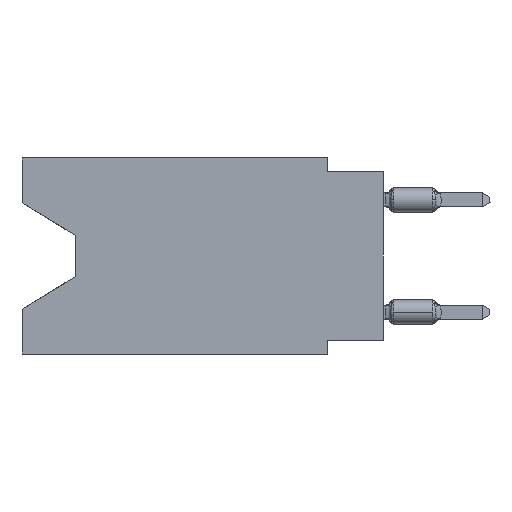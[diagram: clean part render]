
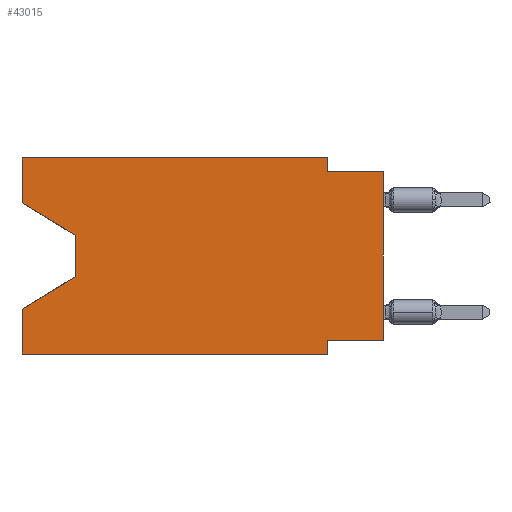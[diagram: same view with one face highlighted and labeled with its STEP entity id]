
A CAD part, left-side view. The second image highlights one B-rep face of the part: STEP entity #43015.
In plain terms, the highlighted planar face has unit normal (-1, 0, 0).
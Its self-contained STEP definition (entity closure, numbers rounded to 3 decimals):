
#37 = VERTEX_POINT ( 'NONE', #25711 ) ;
#702 = CARTESIAN_POINT ( 'NONE',  ( 0., 0., -8.255 ) ) ;
#1206 = EDGE_CURVE ( 'NONE', #21549, #45373, #19123, .T. ) ;
#2084 = PLANE ( 'NONE',  #38290 ) ;
#3101 = EDGE_CURVE ( 'NONE', #45373, #39737, #10770, .T. ) ;
#3219 = CARTESIAN_POINT ( 'NONE',  ( 0., 0., 0. ) ) ;
#4158 = CARTESIAN_POINT ( 'NONE',  ( 0., 16.383, -8.89 ) ) ;
#5878 = ORIENTED_EDGE ( 'NONE', *, *, #19402, .F. ) ;
#6076 = CARTESIAN_POINT ( 'NONE',  ( 0., 0., -0.635 ) ) ;
#7157 = ORIENTED_EDGE ( 'NONE', *, *, #35518, .T. ) ;
#7314 = CARTESIAN_POINT ( 'NONE',  ( 0., 16.383, 0. ) ) ;
#7363 = VECTOR ( 'NONE', #28769, 1000. ) ;
#8396 = DIRECTION ( 'NONE',  ( 0., 1., 0. ) ) ;
#8621 = LINE ( 'NONE', #32381, #10604 ) ;
#9791 = VECTOR ( 'NONE', #45495, 1000. ) ;
#9965 = DIRECTION ( 'NONE',  ( 0., -1., 0. ) ) ;
#10604 = VECTOR ( 'NONE', #8396, 1000. ) ;
#10770 = LINE ( 'NONE', #7314, #21943 ) ;
#11464 = EDGE_CURVE ( 'NONE', #42902, #37655, #41556, .T. ) ;
#12066 = ORIENTED_EDGE ( 'NONE', *, *, #20796, .T. ) ;
#12552 = VERTEX_POINT ( 'NONE', #20235 ) ;
#12775 = VECTOR ( 'NONE', #9965, 1000. ) ;
#13725 = LINE ( 'NONE', #44629, #23203 ) ;
#13886 = ORIENTED_EDGE ( 'NONE', *, *, #19616, .F. ) ;
#14100 = CARTESIAN_POINT ( 'NONE',  ( 0., 2.54, -8.255 ) ) ;
#14379 = ORIENTED_EDGE ( 'NONE', *, *, #3101, .F. ) ;
#14583 = DIRECTION ( 'NONE',  ( 0., 0., -1. ) ) ;
#15799 = LINE ( 'NONE', #19950, #31685 ) ;
#16766 = VECTOR ( 'NONE', #27996, 1000. ) ;
#17135 = CARTESIAN_POINT ( 'NONE',  ( 0., 2.54, -0.635 ) ) ;
#17809 = CARTESIAN_POINT ( 'NONE',  ( 0., 16.383, -8.89 ) ) ;
#18861 = CARTESIAN_POINT ( 'NONE',  ( 0., 16.383, -2.038 ) ) ;
#19123 = LINE ( 'NONE', #21899, #45384 ) ;
#19136 = FACE_OUTER_BOUND ( 'NONE', #28812, .T. ) ;
#19402 = EDGE_CURVE ( 'NONE', #19554, #37, #30507, .T. ) ;
#19421 = CARTESIAN_POINT ( 'NONE',  ( 0., 16.383, -6.852 ) ) ;
#19554 = VERTEX_POINT ( 'NONE', #17135 ) ;
#19589 = CARTESIAN_POINT ( 'NONE',  ( 0., 16.383, 0. ) ) ;
#19616 = EDGE_CURVE ( 'NONE', #24701, #37655, #31420, .T. ) ;
#19875 = VERTEX_POINT ( 'NONE', #19421 ) ;
#19950 = CARTESIAN_POINT ( 'NONE',  ( 0., 2.54, 0. ) ) ;
#20235 = CARTESIAN_POINT ( 'NONE',  ( 0., 13.97, -5.385 ) ) ;
#20460 = EDGE_CURVE ( 'NONE', #30813, #24701, #8621, .T. ) ;
#20515 = LINE ( 'NONE', #3219, #26994 ) ;
#20522 = ORIENTED_EDGE ( 'NONE', *, *, #22407, .T. ) ;
#20660 = CARTESIAN_POINT ( 'NONE',  ( 0., 16.383, -2.038 ) ) ;
#20796 = EDGE_CURVE ( 'NONE', #35473, #12552, #35106, .T. ) ;
#21198 = DIRECTION ( 'NONE',  ( 0., 0., 1. ) ) ;
#21534 = EDGE_CURVE ( 'NONE', #12552, #19875, #13725, .T. ) ;
#21549 = VERTEX_POINT ( 'NONE', #20660 ) ;
#21772 = CARTESIAN_POINT ( 'NONE',  ( 0., 16.383, 0. ) ) ;
#21899 = CARTESIAN_POINT ( 'NONE',  ( 0., 16.383, 0. ) ) ;
#21943 = VECTOR ( 'NONE', #42594, 1000. ) ;
#22407 = EDGE_CURVE ( 'NONE', #21549, #35473, #39629, .T. ) ;
#23049 = EDGE_CURVE ( 'NONE', #39737, #19554, #15799, .T. ) ;
#23203 = VECTOR ( 'NONE', #34251, 1000. ) ;
#24701 = VERTEX_POINT ( 'NONE', #14100 ) ;
#25711 = CARTESIAN_POINT ( 'NONE',  ( 0., 0., -0.635 ) ) ;
#26224 = CARTESIAN_POINT ( 'NONE',  ( 0., 2.54, 0. ) ) ;
#26994 = VECTOR ( 'NONE', #21198, 1000. ) ;
#27373 = ORIENTED_EDGE ( 'NONE', *, *, #21534, .T. ) ;
#27996 = DIRECTION ( 'NONE',  ( 0., 0., 1. ) ) ;
#28174 = CARTESIAN_POINT ( 'NONE',  ( 0., 13.97, -3.505 ) ) ;
#28769 = DIRECTION ( 'NONE',  ( 0., -0.855, -0.519 ) ) ;
#28812 = EDGE_LOOP ( 'NONE', ( #20522, #12066, #27373, #37714, #35140, #13886, #36072, #7157, #5878, #37932, #14379, #31043 ) ) ;
#29260 = DIRECTION ( 'NONE',  ( 0., 0., 1. ) ) ;
#29732 = VECTOR ( 'NONE', #14583, 1000. ) ;
#30182 = DIRECTION ( 'NONE',  ( 0., 0., -1. ) ) ;
#30507 = LINE ( 'NONE', #6076, #41454 ) ;
#30813 = VERTEX_POINT ( 'NONE', #702 ) ;
#31043 = ORIENTED_EDGE ( 'NONE', *, *, #1206, .F. ) ;
#31420 = LINE ( 'NONE', #39266, #9791 ) ;
#31685 = VECTOR ( 'NONE', #34005, 1000. ) ;
#31907 = CARTESIAN_POINT ( 'NONE',  ( 0., 2.54, -8.89 ) ) ;
#32381 = CARTESIAN_POINT ( 'NONE',  ( 0., 0., -8.255 ) ) ;
#33194 = DIRECTION ( 'NONE',  ( 1., 0., 0. ) ) ;
#33208 = CARTESIAN_POINT ( 'NONE',  ( 0., 16.383, 0. ) ) ;
#33900 = CARTESIAN_POINT ( 'NONE',  ( 0., 13.97, -3.505 ) ) ;
#34005 = DIRECTION ( 'NONE',  ( 0., 0., -1. ) ) ;
#34210 = DIRECTION ( 'NONE',  ( 0., -1., 0. ) ) ;
#34251 = DIRECTION ( 'NONE',  ( 0., 0.855, -0.519 ) ) ;
#35106 = LINE ( 'NONE', #28174, #29732 ) ;
#35140 = ORIENTED_EDGE ( 'NONE', *, *, #11464, .T. ) ;
#35473 = VERTEX_POINT ( 'NONE', #33900 ) ;
#35518 = EDGE_CURVE ( 'NONE', #30813, #37, #20515, .T. ) ;
#36072 = ORIENTED_EDGE ( 'NONE', *, *, #20460, .F. ) ;
#36427 = EDGE_CURVE ( 'NONE', #42902, #19875, #42519, .T. ) ;
#37655 = VERTEX_POINT ( 'NONE', #31907 ) ;
#37714 = ORIENTED_EDGE ( 'NONE', *, *, #36427, .F. ) ;
#37932 = ORIENTED_EDGE ( 'NONE', *, *, #23049, .F. ) ;
#38290 = AXIS2_PLACEMENT_3D ( 'NONE', #19589, #33194, #30182 ) ;
#39266 = CARTESIAN_POINT ( 'NONE',  ( 0., 2.54, -8.89 ) ) ;
#39629 = LINE ( 'NONE', #18861, #7363 ) ;
#39737 = VERTEX_POINT ( 'NONE', #26224 ) ;
#41454 = VECTOR ( 'NONE', #34210, 1000. ) ;
#41556 = LINE ( 'NONE', #17809, #12775 ) ;
#42519 = LINE ( 'NONE', #21772, #16766 ) ;
#42594 = DIRECTION ( 'NONE',  ( 0., -1., 0. ) ) ;
#42902 = VERTEX_POINT ( 'NONE', #4158 ) ;
#43015 = ADVANCED_FACE ( 'NONE', ( #19136 ), #2084, .F. ) ;
#44629 = CARTESIAN_POINT ( 'NONE',  ( 0., 13.97, -5.385 ) ) ;
#45373 = VERTEX_POINT ( 'NONE', #33208 ) ;
#45384 = VECTOR ( 'NONE', #29260, 1000. ) ;
#45495 = DIRECTION ( 'NONE',  ( 0., 0., -1. ) ) ;
